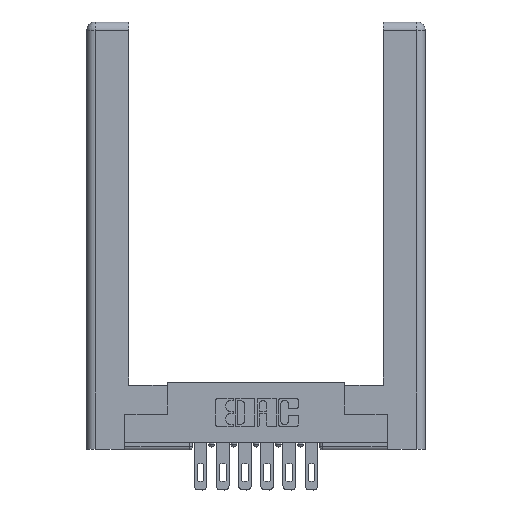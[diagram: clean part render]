
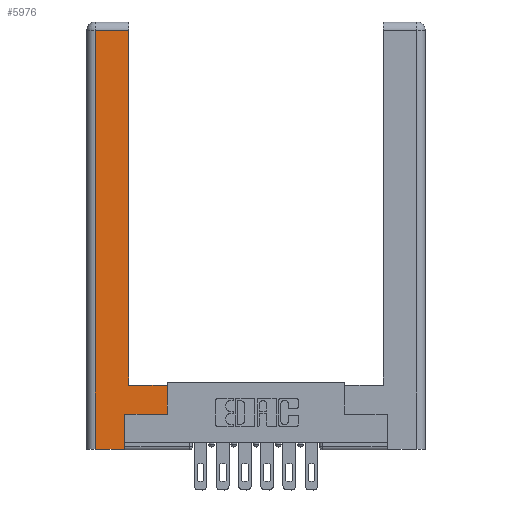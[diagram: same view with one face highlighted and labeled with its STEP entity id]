
A CAD part, top view. The second image highlights one B-rep face of the part: STEP entity #5976.
In plain terms, the highlighted planar face has unit normal (0, 0, 1).
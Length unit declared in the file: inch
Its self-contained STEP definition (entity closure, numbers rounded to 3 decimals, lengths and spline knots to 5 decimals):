
#8 = EDGE_CURVE ( 'NONE', #3507, #10676, #743, .T. ) ;
#208 = CARTESIAN_POINT ( 'NONE',  ( 0.265, 0.245, 0. ) ) ;
#265 = LINE ( 'NONE', #11613, #3457 ) ;
#684 = VECTOR ( 'NONE', #12346, 39.37008 ) ;
#743 = LINE ( 'NONE', #7521, #4821 ) ;
#835 = CARTESIAN_POINT ( 'NONE',  ( 0.265, 0., 0. ) ) ;
#951 = EDGE_CURVE ( 'NONE', #1633, #9101, #265, .T. ) ;
#1233 = DIRECTION ( 'NONE',  ( 0., 1., 0. ) ) ;
#1500 = DIRECTION ( 'NONE',  ( 0., 0., -1. ) ) ;
#1533 = CARTESIAN_POINT ( 'NONE',  ( 0.0615, 2.94, 0. ) ) ;
#1623 = CARTESIAN_POINT ( 'NONE',  ( 0., 0., 0. ) ) ;
#1633 = VERTEX_POINT ( 'NONE', #4153 ) ;
#1659 = EDGE_CURVE ( 'NONE', #9788, #2181, #8025, .T. ) ;
#1691 = VERTEX_POINT ( 'NONE', #8955 ) ;
#1746 = EDGE_CURVE ( 'NONE', #9101, #9788, #11285, .T. ) ;
#2017 = VECTOR ( 'NONE', #10310, 39.37008 ) ;
#2181 = VERTEX_POINT ( 'NONE', #4202 ) ;
#2749 = CARTESIAN_POINT ( 'NONE',  ( 0.565, 0.245, 0. ) ) ;
#2879 = VECTOR ( 'NONE', #8894, 39.37008 ) ;
#3070 = CARTESIAN_POINT ( 'NONE',  ( 0.295, 0.45, 0. ) ) ;
#3329 = CARTESIAN_POINT ( 'NONE',  ( 0.565, 0.45, 0. ) ) ;
#3457 = VECTOR ( 'NONE', #5954, 39.37008 ) ;
#3507 = VERTEX_POINT ( 'NONE', #208 ) ;
#3611 = CARTESIAN_POINT ( 'NONE',  ( 0.295, 2.94, 0. ) ) ;
#3793 = VECTOR ( 'NONE', #1233, 39.37008 ) ;
#4153 = CARTESIAN_POINT ( 'NONE',  ( 0.565, 0.45, 0. ) ) ;
#4163 = AXIS2_PLACEMENT_3D ( 'NONE', #1623, #1500, #6214 ) ;
#4202 = CARTESIAN_POINT ( 'NONE',  ( 0.0615, 2.94, 0. ) ) ;
#4242 = PLANE ( 'NONE',  #4163 ) ;
#4307 = ORIENTED_EDGE ( 'NONE', *, *, #10620, .T. ) ;
#4414 = VERTEX_POINT ( 'NONE', #835 ) ;
#4431 = FACE_OUTER_BOUND ( 'NONE', #12070, .T. ) ;
#4728 = ORIENTED_EDGE ( 'NONE', *, *, #1746, .T. ) ;
#4821 = VECTOR ( 'NONE', #8516, 39.37008 ) ;
#4825 = CARTESIAN_POINT ( 'NONE',  ( 0.265, 0.245, 0. ) ) ;
#4876 = EDGE_CURVE ( 'NONE', #1691, #4414, #10858, .T. ) ;
#4981 = LINE ( 'NONE', #3329, #3793 ) ;
#5954 = DIRECTION ( 'NONE',  ( -1., 0., 0. ) ) ;
#5976 = ADVANCED_FACE ( 'NONE', ( #4431 ), #4242, .F. ) ;
#6214 = DIRECTION ( 'NONE',  ( -1., 0., 0. ) ) ;
#6550 = ORIENTED_EDGE ( 'NONE', *, *, #951, .T. ) ;
#6560 = CARTESIAN_POINT ( 'NONE',  ( 0.295, 3., 0. ) ) ;
#7228 = EDGE_CURVE ( 'NONE', #2181, #1691, #7411, .T. ) ;
#7411 = LINE ( 'NONE', #10891, #2017 ) ;
#7521 = CARTESIAN_POINT ( 'NONE',  ( 0.565, 0.245, 0. ) ) ;
#7762 = VECTOR ( 'NONE', #11791, 39.37008 ) ;
#8025 = LINE ( 'NONE', #1533, #2879 ) ;
#8516 = DIRECTION ( 'NONE',  ( 1., 0., 0. ) ) ;
#8669 = DIRECTION ( 'NONE',  ( 0., 1., 0. ) ) ;
#8836 = CARTESIAN_POINT ( 'NONE',  ( 0.265, 0., 0. ) ) ;
#8894 = DIRECTION ( 'NONE',  ( -1., 0., 0. ) ) ;
#8955 = CARTESIAN_POINT ( 'NONE',  ( 0.0615, 0., 0. ) ) ;
#9101 = VERTEX_POINT ( 'NONE', #3070 ) ;
#9245 = ORIENTED_EDGE ( 'NONE', *, *, #1659, .T. ) ;
#9564 = LINE ( 'NONE', #4825, #11990 ) ;
#9788 = VERTEX_POINT ( 'NONE', #3611 ) ;
#9921 = ORIENTED_EDGE ( 'NONE', *, *, #9951, .T. ) ;
#9951 = EDGE_CURVE ( 'NONE', #10676, #1633, #4981, .T. ) ;
#10310 = DIRECTION ( 'NONE',  ( 0., -1., 0. ) ) ;
#10402 = ORIENTED_EDGE ( 'NONE', *, *, #4876, .T. ) ;
#10620 = EDGE_CURVE ( 'NONE', #4414, #3507, #9564, .T. ) ;
#10676 = VERTEX_POINT ( 'NONE', #2749 ) ;
#10858 = LINE ( 'NONE', #8836, #7762 ) ;
#10891 = CARTESIAN_POINT ( 'NONE',  ( 0.0615, 0., 0. ) ) ;
#11285 = LINE ( 'NONE', #6560, #684 ) ;
#11613 = CARTESIAN_POINT ( 'NONE',  ( 0.295, 0.45, 0. ) ) ;
#11791 = DIRECTION ( 'NONE',  ( 1., 0., 0. ) ) ;
#11990 = VECTOR ( 'NONE', #8669, 39.37008 ) ;
#11997 = ORIENTED_EDGE ( 'NONE', *, *, #8, .T. ) ;
#12070 = EDGE_LOOP ( 'NONE', ( #4728, #9245, #12155, #10402, #4307, #11997, #9921, #6550 ) ) ;
#12155 = ORIENTED_EDGE ( 'NONE', *, *, #7228, .T. ) ;
#12346 = DIRECTION ( 'NONE',  ( 0., 1., 0. ) ) ;
